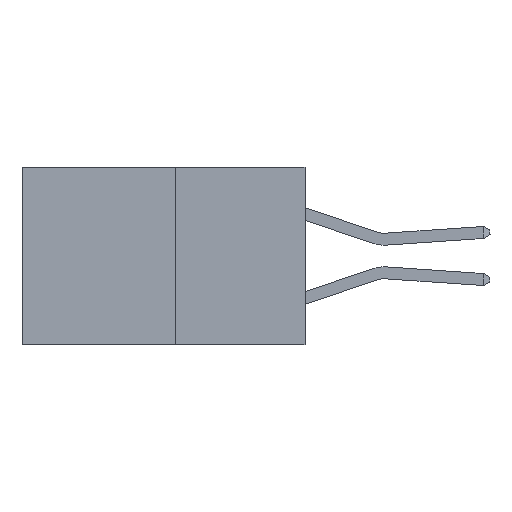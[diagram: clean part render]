
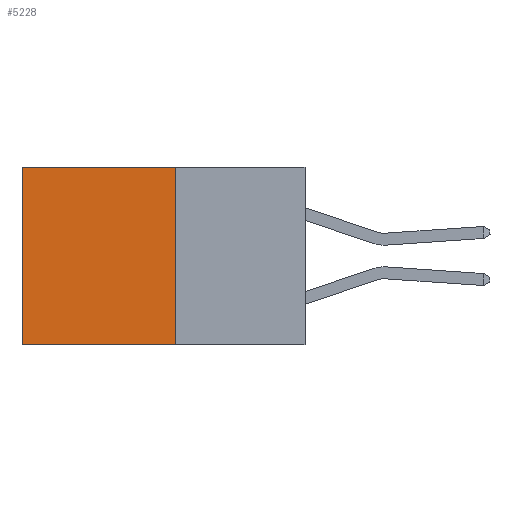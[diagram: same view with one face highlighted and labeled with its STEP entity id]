
A CAD part, left-side view. The second image highlights one B-rep face of the part: STEP entity #5228.
In plain terms, the highlighted planar face has unit normal (-1, 0, 0).
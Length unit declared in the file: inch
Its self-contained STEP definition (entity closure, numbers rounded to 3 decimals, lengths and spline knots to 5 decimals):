
#875 = LINE ( 'NONE', #2160, #2492 ) ;
#1394 = CARTESIAN_POINT ( 'NONE',  ( 0.277, 0.27, -0.37 ) ) ;
#1937 = ORIENTED_EDGE ( 'NONE', *, *, #10005, .F. ) ;
#2140 = DIRECTION ( 'NONE',  ( 0., 1., 0. ) ) ;
#2160 = CARTESIAN_POINT ( 'NONE',  ( 0.277, 0.27, -0.37 ) ) ;
#2427 = EDGE_CURVE ( 'NONE', #7027, #8322, #6611, .T. ) ;
#2492 = VECTOR ( 'NONE', #2871, 39.37008 ) ;
#2543 = EDGE_CURVE ( 'NONE', #7027, #3429, #875, .T. ) ;
#2649 = FACE_OUTER_BOUND ( 'NONE', #3187, .T. ) ;
#2720 = LINE ( 'NONE', #1394, #8743 ) ;
#2871 = DIRECTION ( 'NONE',  ( 0., 0., -1. ) ) ;
#3187 = EDGE_LOOP ( 'NONE', ( #3542, #1937, #9182, #4154 ) ) ;
#3334 = EDGE_CURVE ( 'NONE', #8322, #7496, #5557, .T. ) ;
#3356 = DIRECTION ( 'NONE',  ( 0., 1., 0. ) ) ;
#3429 = VERTEX_POINT ( 'NONE', #9861 ) ;
#3542 = ORIENTED_EDGE ( 'NONE', *, *, #3334, .T. ) ;
#3637 = CARTESIAN_POINT ( 'NONE',  ( 0.277, 0.27, 0. ) ) ;
#4154 = ORIENTED_EDGE ( 'NONE', *, *, #2427, .T. ) ;
#5228 = ADVANCED_FACE ( 'NONE', ( #2649 ), #9722, .F. ) ;
#5514 = CARTESIAN_POINT ( 'NONE',  ( 0.277, 0.27, 0. ) ) ;
#5557 = LINE ( 'NONE', #9396, #9405 ) ;
#5624 = CARTESIAN_POINT ( 'NONE',  ( 0.277, 0.59, 0. ) ) ;
#6116 = DIRECTION ( 'NONE',  ( 0., 0., -1. ) ) ;
#6611 = LINE ( 'NONE', #3637, #8643 ) ;
#7027 = VERTEX_POINT ( 'NONE', #5514 ) ;
#7070 = AXIS2_PLACEMENT_3D ( 'NONE', #8535, #8198, #8147 ) ;
#7496 = VERTEX_POINT ( 'NONE', #9439 ) ;
#8147 = DIRECTION ( 'NONE',  ( 0., 0., -1. ) ) ;
#8198 = DIRECTION ( 'NONE',  ( 1., 0., 0. ) ) ;
#8322 = VERTEX_POINT ( 'NONE', #5624 ) ;
#8535 = CARTESIAN_POINT ( 'NONE',  ( 0.277, 0.27, -0.37 ) ) ;
#8643 = VECTOR ( 'NONE', #3356, 39.37008 ) ;
#8743 = VECTOR ( 'NONE', #2140, 39.37008 ) ;
#9182 = ORIENTED_EDGE ( 'NONE', *, *, #2543, .F. ) ;
#9396 = CARTESIAN_POINT ( 'NONE',  ( 0.277, 0.59, -0.37 ) ) ;
#9405 = VECTOR ( 'NONE', #6116, 39.37008 ) ;
#9439 = CARTESIAN_POINT ( 'NONE',  ( 0.277, 0.59, -0.37 ) ) ;
#9722 = PLANE ( 'NONE',  #7070 ) ;
#9861 = CARTESIAN_POINT ( 'NONE',  ( 0.277, 0.27, -0.37 ) ) ;
#10005 = EDGE_CURVE ( 'NONE', #3429, #7496, #2720, .T. ) ;
